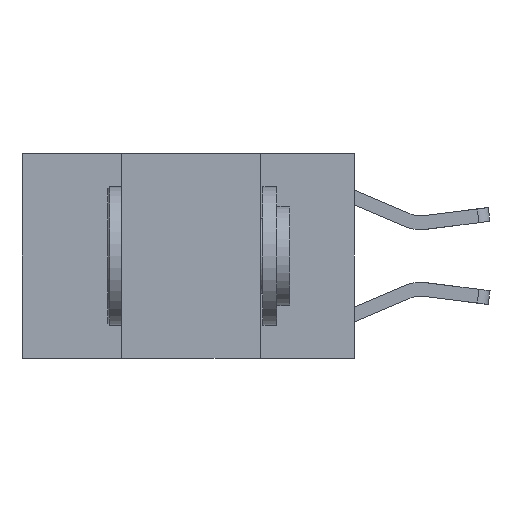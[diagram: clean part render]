
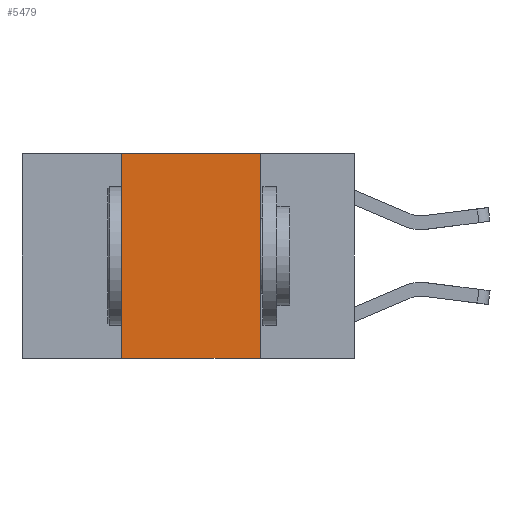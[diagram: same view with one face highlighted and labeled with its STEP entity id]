
A CAD part, left-side view. The second image highlights one B-rep face of the part: STEP entity #5479.
In plain terms, the highlighted planar face has unit normal (-1, 0, 0).
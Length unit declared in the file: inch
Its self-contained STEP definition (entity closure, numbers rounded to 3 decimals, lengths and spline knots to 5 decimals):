
#146 = CARTESIAN_POINT ( 'NONE',  ( 0., 0.6, 0. ) ) ;
#256 = EDGE_CURVE ( 'NONE', #3302, #2457, #6418, .T. ) ;
#479 = EDGE_LOOP ( 'NONE', ( #12089, #7013, #3315, #10603 ) ) ;
#677 = CARTESIAN_POINT ( 'NONE',  ( 0., 0.42, -0.37 ) ) ;
#828 = CARTESIAN_POINT ( 'NONE',  ( 0., 0.6, -0.37 ) ) ;
#1045 = EDGE_CURVE ( 'NONE', #2457, #4703, #3819, .T. ) ;
#1427 = CARTESIAN_POINT ( 'NONE',  ( 0., 0.17, 0. ) ) ;
#1481 = CARTESIAN_POINT ( 'NONE',  ( 0., 0.6, 0. ) ) ;
#1855 = VECTOR ( 'NONE', #11772, 39.37008 ) ;
#2457 = VERTEX_POINT ( 'NONE', #5139 ) ;
#3302 = VERTEX_POINT ( 'NONE', #677 ) ;
#3315 = ORIENTED_EDGE ( 'NONE', *, *, #256, .F. ) ;
#3819 = LINE ( 'NONE', #1481, #1855 ) ;
#3965 = VERTEX_POINT ( 'NONE', #6329 ) ;
#4703 = VERTEX_POINT ( 'NONE', #11903 ) ;
#5139 = CARTESIAN_POINT ( 'NONE',  ( 0., 0.42, 0. ) ) ;
#5216 = AXIS2_PLACEMENT_3D ( 'NONE', #146, #6186, #10235 ) ;
#5437 = CARTESIAN_POINT ( 'NONE',  ( 0., 0.42, 0. ) ) ;
#5479 = ADVANCED_FACE ( 'NONE', ( #6121 ), #9104, .F. ) ;
#5772 = DIRECTION ( 'NONE',  ( 0., -1., 0. ) ) ;
#6121 = FACE_OUTER_BOUND ( 'NONE', #479, .T. ) ;
#6186 = DIRECTION ( 'NONE',  ( 1., 0., 0. ) ) ;
#6329 = CARTESIAN_POINT ( 'NONE',  ( 0., 0.17, -0.37 ) ) ;
#6334 = VECTOR ( 'NONE', #5772, 39.37008 ) ;
#6418 = LINE ( 'NONE', #5437, #8995 ) ;
#6726 = VECTOR ( 'NONE', #10400, 39.37008 ) ;
#7013 = ORIENTED_EDGE ( 'NONE', *, *, #1045, .F. ) ;
#7533 = EDGE_CURVE ( 'NONE', #4703, #3965, #8309, .T. ) ;
#7848 = LINE ( 'NONE', #828, #6334 ) ;
#8291 = DIRECTION ( 'NONE',  ( 0., 0., 1. ) ) ;
#8309 = LINE ( 'NONE', #1427, #6726 ) ;
#8995 = VECTOR ( 'NONE', #8291, 39.37008 ) ;
#9104 = PLANE ( 'NONE',  #5216 ) ;
#10235 = DIRECTION ( 'NONE',  ( 0., 0., -1. ) ) ;
#10400 = DIRECTION ( 'NONE',  ( 0., 0., -1. ) ) ;
#10603 = ORIENTED_EDGE ( 'NONE', *, *, #12363, .T. ) ;
#11772 = DIRECTION ( 'NONE',  ( 0., -1., 0. ) ) ;
#11903 = CARTESIAN_POINT ( 'NONE',  ( 0., 0.17, 0. ) ) ;
#12089 = ORIENTED_EDGE ( 'NONE', *, *, #7533, .F. ) ;
#12363 = EDGE_CURVE ( 'NONE', #3302, #3965, #7848, .T. ) ;
